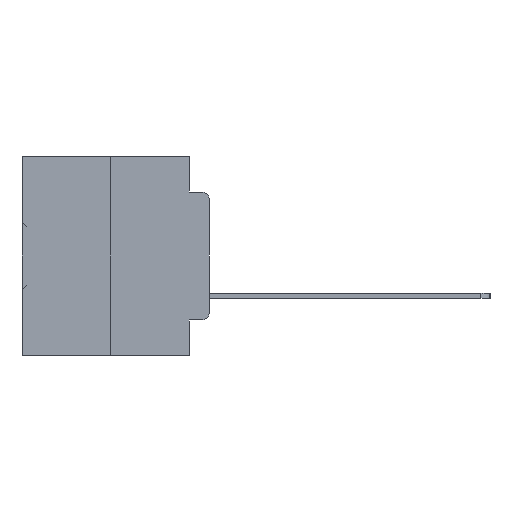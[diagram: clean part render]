
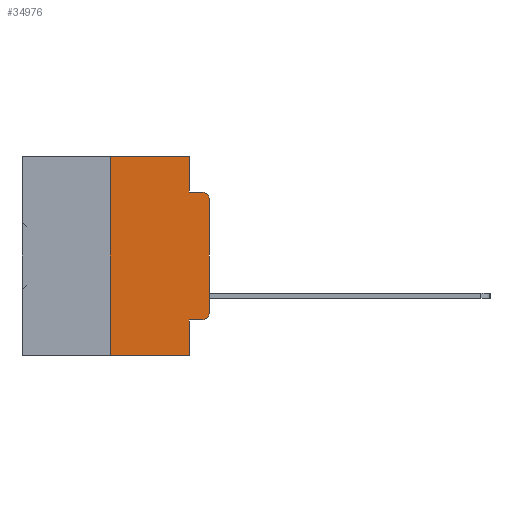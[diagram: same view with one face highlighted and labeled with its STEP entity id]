
A CAD part, left-side view. The second image highlights one B-rep face of the part: STEP entity #34976.
In plain terms, the highlighted planar face has unit normal (-1, 0, 0).
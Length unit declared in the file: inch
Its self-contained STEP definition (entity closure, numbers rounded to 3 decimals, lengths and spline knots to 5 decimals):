
#307 = VERTEX_POINT ( 'NONE', #26127 ) ;
#514 = EDGE_CURVE ( 'NONE', #21072, #11292, #36972, .T. ) ;
#603 = VERTEX_POINT ( 'NONE', #13724 ) ;
#700 = ORIENTED_EDGE ( 'NONE', *, *, #6317, .T. ) ;
#726 = VERTEX_POINT ( 'NONE', #9609 ) ;
#1653 = EDGE_LOOP ( 'NONE', ( #700, #26532, #11646, #25710, #28336, #12577, #13996, #20390, #11299, #8132 ) ) ;
#2565 = VERTEX_POINT ( 'NONE', #31352 ) ;
#3248 = VECTOR ( 'NONE', #9826, 39.37008 ) ;
#4376 = EDGE_CURVE ( 'NONE', #24503, #11292, #19348, .T. ) ;
#5035 = CARTESIAN_POINT ( 'NONE',  ( 0., 0.25, 0. ) ) ;
#5316 = DIRECTION ( 'NONE',  ( 0., -1., 0. ) ) ;
#6252 = CARTESIAN_POINT ( 'NONE',  ( 0., 0.473, -0.5 ) ) ;
#6273 = CARTESIAN_POINT ( 'NONE',  ( 0., 0., -0.1085 ) ) ;
#6317 = EDGE_CURVE ( 'NONE', #18631, #24503, #21983, .T. ) ;
#6355 = CARTESIAN_POINT ( 'NONE',  ( 0., 0.051, -0.0885 ) ) ;
#6857 = CARTESIAN_POINT ( 'NONE',  ( 0., 0.473, 0. ) ) ;
#7400 = LINE ( 'NONE', #5035, #21054 ) ;
#7721 = CARTESIAN_POINT ( 'NONE',  ( 0., 0.051, 0. ) ) ;
#8132 = ORIENTED_EDGE ( 'NONE', *, *, #24593, .T. ) ;
#9609 = CARTESIAN_POINT ( 'NONE',  ( 0., 0.25, -0.5 ) ) ;
#9612 = CARTESIAN_POINT ( 'NONE',  ( 0., 0.02, -0.3915 ) ) ;
#9826 = DIRECTION ( 'NONE',  ( 0., -1., 0. ) ) ;
#9882 = VECTOR ( 'NONE', #26649, 39.37008 ) ;
#10324 = CARTESIAN_POINT ( 'NONE',  ( 0., 0.051, -0.0885 ) ) ;
#10466 = VECTOR ( 'NONE', #11882, 39.37008 ) ;
#10644 = DIRECTION ( 'NONE',  ( 0., 0., -1. ) ) ;
#10993 = DIRECTION ( 'NONE',  ( 1., 0., 0. ) ) ;
#11292 = VERTEX_POINT ( 'NONE', #17363 ) ;
#11299 = ORIENTED_EDGE ( 'NONE', *, *, #28366, .T. ) ;
#11580 = AXIS2_PLACEMENT_3D ( 'NONE', #9612, #29715, #12519 ) ;
#11646 = ORIENTED_EDGE ( 'NONE', *, *, #514, .F. ) ;
#11697 = LINE ( 'NONE', #6252, #9882 ) ;
#11882 = DIRECTION ( 'NONE',  ( 0., -1., 0. ) ) ;
#11897 = LINE ( 'NONE', #6857, #3248 ) ;
#11950 = CARTESIAN_POINT ( 'NONE',  ( 0., 0.02, -0.1085 ) ) ;
#12519 = DIRECTION ( 'NONE',  ( 0., 0., -1. ) ) ;
#12577 = ORIENTED_EDGE ( 'NONE', *, *, #32110, .F. ) ;
#13086 = LINE ( 'NONE', #25497, #19940 ) ;
#13724 = CARTESIAN_POINT ( 'NONE',  ( 0., 0.051, 0. ) ) ;
#13996 = ORIENTED_EDGE ( 'NONE', *, *, #22134, .T. ) ;
#14883 = DIRECTION ( 'NONE',  ( 0., 0., -1. ) ) ;
#16654 = DIRECTION ( 'NONE',  ( 0., 0., 1. ) ) ;
#17095 = VERTEX_POINT ( 'NONE', #21357 ) ;
#17363 = CARTESIAN_POINT ( 'NONE',  ( 0., 0.02, -0.0885 ) ) ;
#18198 = LINE ( 'NONE', #31937, #10466 ) ;
#18631 = VERTEX_POINT ( 'NONE', #26400 ) ;
#18715 = VERTEX_POINT ( 'NONE', #26638 ) ;
#19348 = CIRCLE ( 'NONE', #26543, 0.02 ) ;
#19639 = CARTESIAN_POINT ( 'NONE',  ( 0., 0.473, 0. ) ) ;
#19940 = VECTOR ( 'NONE', #33981, 39.37008 ) ;
#20390 = ORIENTED_EDGE ( 'NONE', *, *, #30239, .F. ) ;
#21054 = VECTOR ( 'NONE', #16654, 39.37008 ) ;
#21072 = VERTEX_POINT ( 'NONE', #10324 ) ;
#21357 = CARTESIAN_POINT ( 'NONE',  ( 0., 0.051, -0.5 ) ) ;
#21684 = AXIS2_PLACEMENT_3D ( 'NONE', #19639, #10993, #31052 ) ;
#21972 = VECTOR ( 'NONE', #5316, 39.37008 ) ;
#21983 = LINE ( 'NONE', #35579, #36093 ) ;
#22134 = EDGE_CURVE ( 'NONE', #726, #17095, #11697, .T. ) ;
#22169 = VECTOR ( 'NONE', #10644, 39.37008 ) ;
#23077 = LINE ( 'NONE', #7721, #22169 ) ;
#24503 = VERTEX_POINT ( 'NONE', #6273 ) ;
#24593 = EDGE_CURVE ( 'NONE', #18715, #18631, #28215, .T. ) ;
#25497 = CARTESIAN_POINT ( 'NONE',  ( 0., 0.051, 0. ) ) ;
#25710 = ORIENTED_EDGE ( 'NONE', *, *, #35897, .F. ) ;
#26127 = CARTESIAN_POINT ( 'NONE',  ( 0., 0.051, -0.4115 ) ) ;
#26400 = CARTESIAN_POINT ( 'NONE',  ( 0., 0., -0.3915 ) ) ;
#26532 = ORIENTED_EDGE ( 'NONE', *, *, #4376, .T. ) ;
#26543 = AXIS2_PLACEMENT_3D ( 'NONE', #11950, #31998, #14883 ) ;
#26638 = CARTESIAN_POINT ( 'NONE',  ( 0., 0.02, -0.4115 ) ) ;
#26649 = DIRECTION ( 'NONE',  ( 0., -1., 0. ) ) ;
#27271 = EDGE_CURVE ( 'NONE', #2565, #603, #11897, .T. ) ;
#28215 = CIRCLE ( 'NONE', #11580, 0.02 ) ;
#28336 = ORIENTED_EDGE ( 'NONE', *, *, #27271, .F. ) ;
#28366 = EDGE_CURVE ( 'NONE', #307, #18715, #18198, .T. ) ;
#29715 = DIRECTION ( 'NONE',  ( -1., 0., 0. ) ) ;
#30239 = EDGE_CURVE ( 'NONE', #307, #17095, #13086, .T. ) ;
#30931 = PLANE ( 'NONE',  #21684 ) ;
#31052 = DIRECTION ( 'NONE',  ( 0., 0., -1. ) ) ;
#31352 = CARTESIAN_POINT ( 'NONE',  ( 0., 0.25, 0. ) ) ;
#31937 = CARTESIAN_POINT ( 'NONE',  ( 0., 0.051, -0.4115 ) ) ;
#31998 = DIRECTION ( 'NONE',  ( -1., 0., 0. ) ) ;
#32110 = EDGE_CURVE ( 'NONE', #726, #2565, #7400, .T. ) ;
#32735 = DIRECTION ( 'NONE',  ( 0., 0., 1. ) ) ;
#33981 = DIRECTION ( 'NONE',  ( 0., 0., -1. ) ) ;
#34187 = FACE_OUTER_BOUND ( 'NONE', #1653, .T. ) ;
#34976 = ADVANCED_FACE ( 'NONE', ( #34187 ), #30931, .F. ) ;
#35579 = CARTESIAN_POINT ( 'NONE',  ( 0., 0., 0. ) ) ;
#35897 = EDGE_CURVE ( 'NONE', #603, #21072, #23077, .T. ) ;
#36093 = VECTOR ( 'NONE', #32735, 39.37008 ) ;
#36972 = LINE ( 'NONE', #6355, #21972 ) ;
